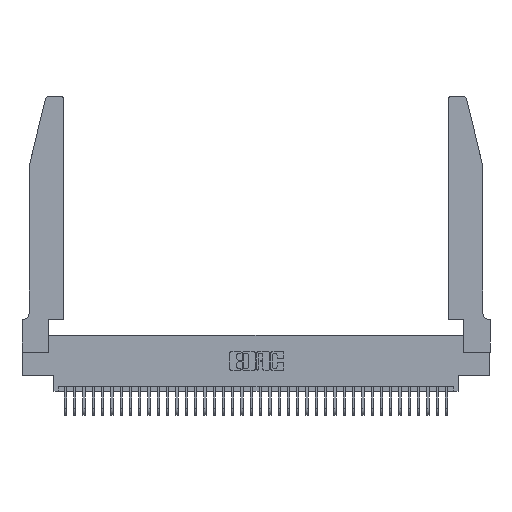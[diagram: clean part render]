
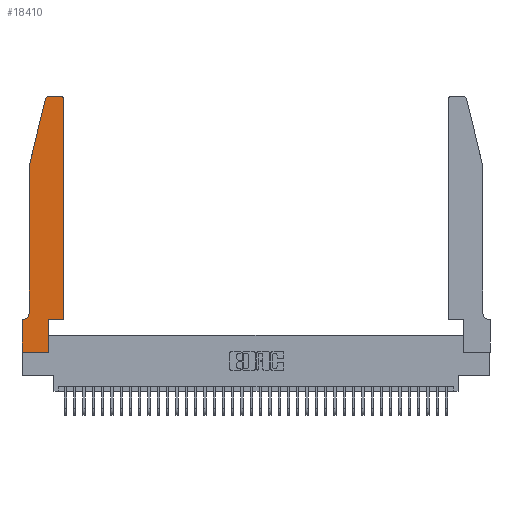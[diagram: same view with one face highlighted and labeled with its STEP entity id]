
A CAD part, top view. The second image highlights one B-rep face of the part: STEP entity #18410.
In plain terms, the highlighted planar face has unit normal (0, 0, 1).
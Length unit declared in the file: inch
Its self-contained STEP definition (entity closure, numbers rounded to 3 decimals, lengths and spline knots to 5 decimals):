
#518 = ORIENTED_EDGE ( 'NONE', *, *, #26552, .T. ) ;
#1655 = VERTEX_POINT ( 'NONE', #30151 ) ;
#1705 = VERTEX_POINT ( 'NONE', #8096 ) ;
#2430 = CARTESIAN_POINT ( 'NONE',  ( 0.284, 2.72, 0.37 ) ) ;
#2715 = VERTEX_POINT ( 'NONE', #30023 ) ;
#2781 = VECTOR ( 'NONE', #13481, 39.37008 ) ;
#2894 = VECTOR ( 'NONE', #9503, 39.37008 ) ;
#3001 = LINE ( 'NONE', #34594, #20574 ) ;
#3176 = CARTESIAN_POINT ( 'NONE',  ( 0.0055, 0.35, 0.37 ) ) ;
#3713 = CARTESIAN_POINT ( 'NONE',  ( 0., 0., 0.37 ) ) ;
#4188 = CIRCLE ( 'NONE', #20425, 0.07 ) ;
#4297 = EDGE_CURVE ( 'NONE', #20550, #1655, #39120, .T. ) ;
#4365 = VERTEX_POINT ( 'NONE', #23140 ) ;
#4379 = PLANE ( 'NONE',  #22298 ) ;
#4625 = VERTEX_POINT ( 'NONE', #22865 ) ;
#5024 = EDGE_CURVE ( 'NONE', #11173, #4625, #18014, .T. ) ;
#5434 = LINE ( 'NONE', #5962, #19677 ) ;
#5679 = ORIENTED_EDGE ( 'NONE', *, *, #25880, .T. ) ;
#5919 = EDGE_CURVE ( 'NONE', #1705, #17948, #3001, .T. ) ;
#5962 = CARTESIAN_POINT ( 'NONE',  ( 0.4505, 0.35, 0.37 ) ) ;
#6244 = DIRECTION ( 'NONE',  ( 1., 0., 0. ) ) ;
#6711 = EDGE_CURVE ( 'NONE', #1655, #1705, #5434, .T. ) ;
#6789 = ORIENTED_EDGE ( 'NONE', *, *, #30204, .T. ) ;
#6793 = DIRECTION ( 'NONE',  ( 0., -1., 0. ) ) ;
#7899 = DIRECTION ( 'NONE',  ( 0., 0., 1. ) ) ;
#8096 = CARTESIAN_POINT ( 'NONE',  ( 0.4505, 0.35, 0.37 ) ) ;
#8392 = CARTESIAN_POINT ( 'NONE',  ( 0.0755, 0.35, 0.37 ) ) ;
#8640 = LINE ( 'NONE', #10009, #2894 ) ;
#9117 = DIRECTION ( 'NONE',  ( 0., 1., 0. ) ) ;
#9364 = EDGE_CURVE ( 'NONE', #30734, #4365, #18091, .T. ) ;
#9503 = DIRECTION ( 'NONE',  ( 1., 0., 0. ) ) ;
#9733 = DIRECTION ( 'NONE',  ( 0., 1., 0. ) ) ;
#9889 = CARTESIAN_POINT ( 'NONE',  ( 0., 0.35, 0.37 ) ) ;
#10009 = CARTESIAN_POINT ( 'NONE',  ( 0., 0., 0.37 ) ) ;
#11173 = VERTEX_POINT ( 'NONE', #12332 ) ;
#11414 = DIRECTION ( 'NONE',  ( -1., 0., 0. ) ) ;
#11562 = ORIENTED_EDGE ( 'NONE', *, *, #5024, .T. ) ;
#12332 = CARTESIAN_POINT ( 'NONE',  ( 0.4205, 2.75, 0.37 ) ) ;
#12714 = CIRCLE ( 'NONE', #39407, 0.03 ) ;
#13317 = ORIENTED_EDGE ( 'NONE', *, *, #4297, .T. ) ;
#13481 = DIRECTION ( 'NONE',  ( -1., 0., 0. ) ) ;
#14792 = DIRECTION ( 'NONE',  ( 0., 0., 1. ) ) ;
#15021 = EDGE_CURVE ( 'NONE', #17948, #11173, #12714, .T. ) ;
#15704 = DIRECTION ( 'NONE',  ( -0.239, -0.971, 0. ) ) ;
#15767 = CIRCLE ( 'NONE', #19245, 0.03 ) ;
#16310 = VERTEX_POINT ( 'NONE', #29196 ) ;
#16776 = DIRECTION ( 'NONE',  ( 0., -1., 0. ) ) ;
#17159 = VERTEX_POINT ( 'NONE', #36623 ) ;
#17911 = FACE_OUTER_BOUND ( 'NONE', #36628, .T. ) ;
#17948 = VERTEX_POINT ( 'NONE', #34583 ) ;
#18014 = LINE ( 'NONE', #31661, #2781 ) ;
#18091 = LINE ( 'NONE', #28432, #28113 ) ;
#18410 = ADVANCED_FACE ( 'NONE', ( #17911 ), #4379, .T. ) ;
#19245 = AXIS2_PLACEMENT_3D ( 'NONE', #2430, #14792, #32956 ) ;
#19282 = DIRECTION ( 'NONE',  ( -1., 0., 0. ) ) ;
#19357 = VECTOR ( 'NONE', #6793, 39.37008 ) ;
#19491 = CARTESIAN_POINT ( 'NONE',  ( 0.4205, 2.72, 0.37 ) ) ;
#19677 = VECTOR ( 'NONE', #29940, 39.37008 ) ;
#19893 = DIRECTION ( 'NONE',  ( 0., 0., 1. ) ) ;
#19980 = EDGE_CURVE ( 'NONE', #4625, #17159, #15767, .T. ) ;
#20425 = AXIS2_PLACEMENT_3D ( 'NONE', #37581, #28514, #19282 ) ;
#20488 = ORIENTED_EDGE ( 'NONE', *, *, #33732, .T. ) ;
#20550 = VERTEX_POINT ( 'NONE', #22071 ) ;
#20574 = VECTOR ( 'NONE', #9733, 39.37008 ) ;
#21034 = ORIENTED_EDGE ( 'NONE', *, *, #6711, .T. ) ;
#21555 = ORIENTED_EDGE ( 'NONE', *, *, #15021, .T. ) ;
#21584 = CARTESIAN_POINT ( 'NONE',  ( 0.0755, 2., 0.37 ) ) ;
#22071 = CARTESIAN_POINT ( 'NONE',  ( 0.2865, 0., 0.37 ) ) ;
#22298 = AXIS2_PLACEMENT_3D ( 'NONE', #9889, #19893, #22699 ) ;
#22699 = DIRECTION ( 'NONE',  ( 1., 0., 0. ) ) ;
#22865 = CARTESIAN_POINT ( 'NONE',  ( 0.284, 2.75, 0.37 ) ) ;
#23140 = CARTESIAN_POINT ( 'NONE',  ( 0.0755, 0.42, 0.37 ) ) ;
#24420 = ORIENTED_EDGE ( 'NONE', *, *, #19980, .T. ) ;
#24760 = VECTOR ( 'NONE', #9117, 39.37008 ) ;
#25880 = EDGE_CURVE ( 'NONE', #4365, #36489, #4188, .T. ) ;
#25895 = VECTOR ( 'NONE', #11414, 39.37008 ) ;
#26492 = EDGE_CURVE ( 'NONE', #17159, #30734, #32295, .T. ) ;
#26552 = EDGE_CURVE ( 'NONE', #16310, #2715, #27511, .T. ) ;
#27244 = ORIENTED_EDGE ( 'NONE', *, *, #5919, .T. ) ;
#27511 = LINE ( 'NONE', #3713, #19357 ) ;
#28113 = VECTOR ( 'NONE', #16776, 39.37008 ) ;
#28432 = CARTESIAN_POINT ( 'NONE',  ( 0.0755, 2., 0.37 ) ) ;
#28514 = DIRECTION ( 'NONE',  ( 0., 0., -1. ) ) ;
#29196 = CARTESIAN_POINT ( 'NONE',  ( 0., 0.35, 0.37 ) ) ;
#29498 = ORIENTED_EDGE ( 'NONE', *, *, #9364, .T. ) ;
#29792 = CARTESIAN_POINT ( 'NONE',  ( 0.0755, 2., 0.37 ) ) ;
#29940 = DIRECTION ( 'NONE',  ( 1., 0., 0. ) ) ;
#30023 = CARTESIAN_POINT ( 'NONE',  ( 0., 0., 0.37 ) ) ;
#30151 = CARTESIAN_POINT ( 'NONE',  ( 0.2865, 0.35, 0.37 ) ) ;
#30204 = EDGE_CURVE ( 'NONE', #2715, #20550, #8640, .T. ) ;
#30734 = VERTEX_POINT ( 'NONE', #29792 ) ;
#31661 = CARTESIAN_POINT ( 'NONE',  ( 0.2605, 2.75, 0.37 ) ) ;
#32295 = LINE ( 'NONE', #21584, #36139 ) ;
#32956 = DIRECTION ( 'NONE',  ( 1., 0., 0. ) ) ;
#33732 = EDGE_CURVE ( 'NONE', #36489, #16310, #34982, .T. ) ;
#34583 = CARTESIAN_POINT ( 'NONE',  ( 0.4505, 2.72, 0.37 ) ) ;
#34594 = CARTESIAN_POINT ( 'NONE',  ( 0.4505, 0.35, 0.37 ) ) ;
#34982 = LINE ( 'NONE', #8392, #25895 ) ;
#35873 = ORIENTED_EDGE ( 'NONE', *, *, #26492, .T. ) ;
#36139 = VECTOR ( 'NONE', #15704, 39.37008 ) ;
#36190 = CARTESIAN_POINT ( 'NONE',  ( 0.2865, 0.35, 0.37 ) ) ;
#36489 = VERTEX_POINT ( 'NONE', #3176 ) ;
#36623 = CARTESIAN_POINT ( 'NONE',  ( 0.25487, 2.72718, 0.37 ) ) ;
#36628 = EDGE_LOOP ( 'NONE', ( #11562, #24420, #35873, #29498, #5679, #20488, #518, #6789, #13317, #21034, #27244, #21555 ) ) ;
#37581 = CARTESIAN_POINT ( 'NONE',  ( 0.0055, 0.42, 0.37 ) ) ;
#39120 = LINE ( 'NONE', #36190, #24760 ) ;
#39407 = AXIS2_PLACEMENT_3D ( 'NONE', #19491, #7899, #6244 ) ;
